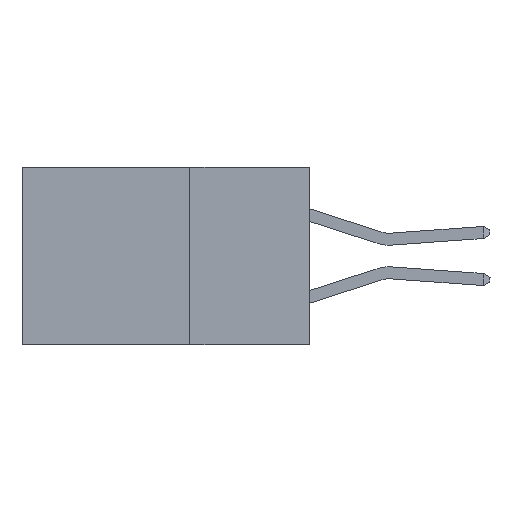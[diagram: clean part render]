
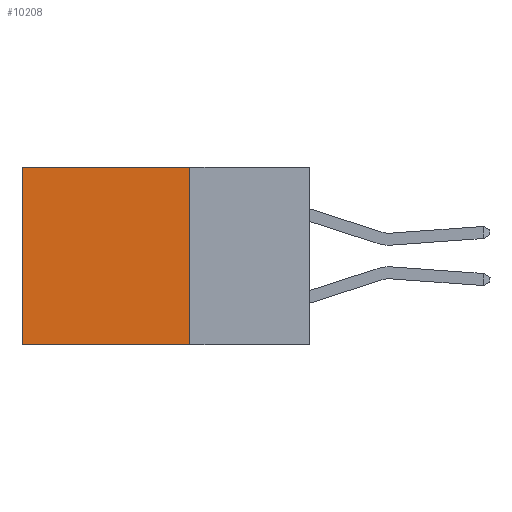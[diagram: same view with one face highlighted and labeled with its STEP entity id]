
A CAD part, left-side view. The second image highlights one B-rep face of the part: STEP entity #10208.
In plain terms, the highlighted planar face has unit normal (-1, 0, 0).
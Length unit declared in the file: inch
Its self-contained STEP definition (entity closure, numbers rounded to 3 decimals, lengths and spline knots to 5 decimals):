
#622 = EDGE_CURVE ( 'NONE', #14337, #13567, #16986, .T. ) ;
#859 = LINE ( 'NONE', #8504, #14944 ) ;
#1113 = PLANE ( 'NONE',  #16007 ) ;
#1326 = CARTESIAN_POINT ( 'NONE',  ( 0.298, 0.6, 0. ) ) ;
#2178 = VECTOR ( 'NONE', #9583, 39.37008 ) ;
#2365 = CARTESIAN_POINT ( 'NONE',  ( 0.298, 0.25, 0. ) ) ;
#2629 = ORIENTED_EDGE ( 'NONE', *, *, #8752, .F. ) ;
#2732 = CARTESIAN_POINT ( 'NONE',  ( 0.298, 0.25, 0. ) ) ;
#3653 = LINE ( 'NONE', #2732, #2178 ) ;
#4042 = VECTOR ( 'NONE', #7560, 39.37008 ) ;
#5300 = VERTEX_POINT ( 'NONE', #10521 ) ;
#6088 = CARTESIAN_POINT ( 'NONE',  ( 0.298, 0.25, 0. ) ) ;
#6202 = CARTESIAN_POINT ( 'NONE',  ( 0.298, 0.25, -0.37 ) ) ;
#6615 = ORIENTED_EDGE ( 'NONE', *, *, #622, .T. ) ;
#6633 = FACE_OUTER_BOUND ( 'NONE', #7570, .T. ) ;
#6840 = DIRECTION ( 'NONE',  ( 0., 0., -1. ) ) ;
#7560 = DIRECTION ( 'NONE',  ( 0., 1., 0. ) ) ;
#7570 = EDGE_LOOP ( 'NONE', ( #6615, #15512, #2629, #17194 ) ) ;
#8504 = CARTESIAN_POINT ( 'NONE',  ( 0.298, 0.25, 0. ) ) ;
#8752 = EDGE_CURVE ( 'NONE', #9932, #5300, #3653, .T. ) ;
#9023 = CARTESIAN_POINT ( 'NONE',  ( 0.298, 0.6, 0. ) ) ;
#9084 = VECTOR ( 'NONE', #6840, 39.37008 ) ;
#9113 = DIRECTION ( 'NONE',  ( 0., 0., -1. ) ) ;
#9583 = DIRECTION ( 'NONE',  ( 0., 0., -1. ) ) ;
#9872 = DIRECTION ( 'NONE',  ( 0., 1., 0. ) ) ;
#9932 = VERTEX_POINT ( 'NONE', #6088 ) ;
#10164 = EDGE_CURVE ( 'NONE', #5300, #13567, #14312, .T. ) ;
#10208 = ADVANCED_FACE ( 'NONE', ( #6633 ), #1113, .F. ) ;
#10521 = CARTESIAN_POINT ( 'NONE',  ( 0.298, 0.25, -0.37 ) ) ;
#11897 = DIRECTION ( 'NONE',  ( 1., 0., 0. ) ) ;
#13567 = VERTEX_POINT ( 'NONE', #17549 ) ;
#14312 = LINE ( 'NONE', #6202, #4042 ) ;
#14337 = VERTEX_POINT ( 'NONE', #9023 ) ;
#14944 = VECTOR ( 'NONE', #9872, 39.37008 ) ;
#15512 = ORIENTED_EDGE ( 'NONE', *, *, #10164, .F. ) ;
#15929 = EDGE_CURVE ( 'NONE', #9932, #14337, #859, .T. ) ;
#16007 = AXIS2_PLACEMENT_3D ( 'NONE', #2365, #11897, #9113 ) ;
#16986 = LINE ( 'NONE', #1326, #9084 ) ;
#17194 = ORIENTED_EDGE ( 'NONE', *, *, #15929, .T. ) ;
#17549 = CARTESIAN_POINT ( 'NONE',  ( 0.298, 0.6, -0.37 ) ) ;
